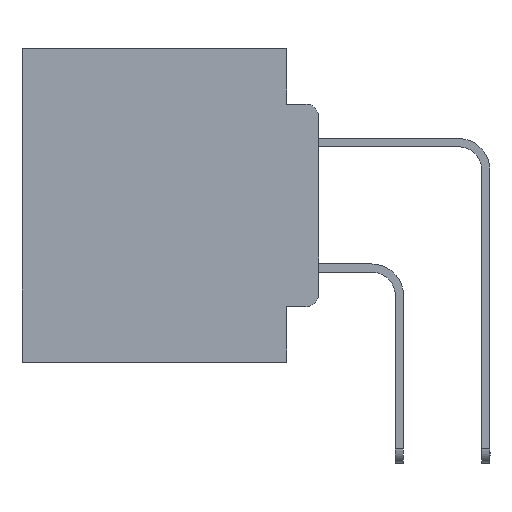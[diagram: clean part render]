
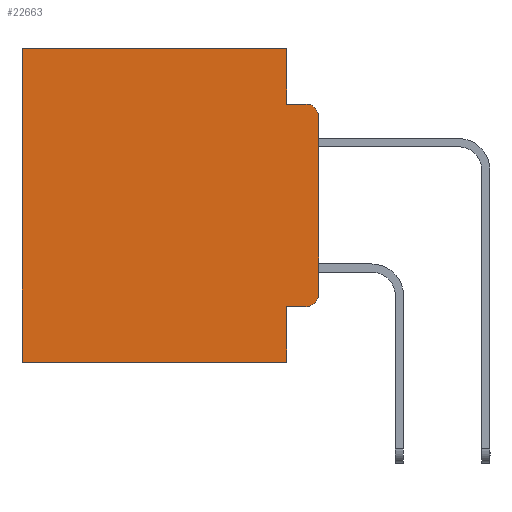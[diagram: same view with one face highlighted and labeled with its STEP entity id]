
A CAD part, left-side view. The second image highlights one B-rep face of the part: STEP entity #22663.
In plain terms, the highlighted planar face has unit normal (-1, 0, 0).
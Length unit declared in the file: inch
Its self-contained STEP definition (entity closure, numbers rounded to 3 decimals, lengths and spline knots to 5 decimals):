
#62 = EDGE_CURVE ( 'NONE', #12514, #3945, #13382, .T. ) ;
#63 = EDGE_LOOP ( 'NONE', ( #21769, #2561, #18959, #17731, #18588, #6089, #12443, #4766, #265, #25057 ) ) ;
#265 = ORIENTED_EDGE ( 'NONE', *, *, #27777, .T. ) ;
#346 = CARTESIAN_POINT ( 'NONE',  ( 0.298, 0.051, 0. ) ) ;
#623 = LINE ( 'NONE', #18278, #24192 ) ;
#1104 = PLANE ( 'NONE',  #4373 ) ;
#1684 = VECTOR ( 'NONE', #17175, 39.37008 ) ;
#1720 = DIRECTION ( 'NONE',  ( -1., 0., 0. ) ) ;
#1902 = LINE ( 'NONE', #10855, #5172 ) ;
#2036 = DIRECTION ( 'NONE',  ( -1., 0., 0. ) ) ;
#2121 = VERTEX_POINT ( 'NONE', #9627 ) ;
#2561 = ORIENTED_EDGE ( 'NONE', *, *, #25646, .T. ) ;
#2617 = EDGE_CURVE ( 'NONE', #12514, #18378, #17990, .T. ) ;
#3945 = VERTEX_POINT ( 'NONE', #20756 ) ;
#4373 = AXIS2_PLACEMENT_3D ( 'NONE', #25403, #14542, #9936 ) ;
#4402 = CARTESIAN_POINT ( 'NONE',  ( 0.298, 0.02, -0.4115 ) ) ;
#4596 = CARTESIAN_POINT ( 'NONE',  ( 0.298, 0.473, 0. ) ) ;
#4766 = ORIENTED_EDGE ( 'NONE', *, *, #17363, .F. ) ;
#5102 = CARTESIAN_POINT ( 'NONE',  ( 0.298, 0.051, -0.0885 ) ) ;
#5162 = CARTESIAN_POINT ( 'NONE',  ( 0.298, 0.051, -0.4115 ) ) ;
#5172 = VECTOR ( 'NONE', #25903, 39.37008 ) ;
#5721 = CIRCLE ( 'NONE', #9902, 0.02 ) ;
#5852 = VECTOR ( 'NONE', #24654, 39.37008 ) ;
#5875 = VECTOR ( 'NONE', #18188, 39.37008 ) ;
#6089 = ORIENTED_EDGE ( 'NONE', *, *, #8888, .T. ) ;
#6342 = CARTESIAN_POINT ( 'NONE',  ( 0.298, 0.02, -0.1085 ) ) ;
#6419 = VECTOR ( 'NONE', #6454, 39.37008 ) ;
#6454 = DIRECTION ( 'NONE',  ( 0., 1., 0. ) ) ;
#6927 = LINE ( 'NONE', #5162, #5875 ) ;
#7237 = LINE ( 'NONE', #7379, #23154 ) ;
#7301 = DIRECTION ( 'NONE',  ( 0., 0., -1. ) ) ;
#7379 = CARTESIAN_POINT ( 'NONE',  ( 0.298, 0., -0.5 ) ) ;
#8370 = CARTESIAN_POINT ( 'NONE',  ( 0.298, 0.051, -0.0885 ) ) ;
#8377 = DIRECTION ( 'NONE',  ( 0., 0., -1. ) ) ;
#8888 = EDGE_CURVE ( 'NONE', #3945, #11539, #23809, .T. ) ;
#9115 = VERTEX_POINT ( 'NONE', #21038 ) ;
#9627 = CARTESIAN_POINT ( 'NONE',  ( 0.298, 0., -0.1085 ) ) ;
#9902 = AXIS2_PLACEMENT_3D ( 'NONE', #13582, #2036, #17627 ) ;
#9936 = DIRECTION ( 'NONE',  ( 0., 0., -1. ) ) ;
#10855 = CARTESIAN_POINT ( 'NONE',  ( 0.298, 0.051, 0. ) ) ;
#10905 = VERTEX_POINT ( 'NONE', #4402 ) ;
#11539 = VERTEX_POINT ( 'NONE', #15780 ) ;
#11843 = VERTEX_POINT ( 'NONE', #24680 ) ;
#12443 = ORIENTED_EDGE ( 'NONE', *, *, #17432, .F. ) ;
#12514 = VERTEX_POINT ( 'NONE', #17100 ) ;
#12809 = CARTESIAN_POINT ( 'NONE',  ( 0.298, 0., 0. ) ) ;
#13382 = LINE ( 'NONE', #12809, #6419 ) ;
#13582 = CARTESIAN_POINT ( 'NONE',  ( 0.298, 0.02, -0.3915 ) ) ;
#14542 = DIRECTION ( 'NONE',  ( 1., 0., 0. ) ) ;
#14545 = VECTOR ( 'NONE', #17297, 39.37008 ) ;
#15626 = DIRECTION ( 'NONE',  ( 0., 1., 0. ) ) ;
#15780 = CARTESIAN_POINT ( 'NONE',  ( 0.298, 0.473, -0.5 ) ) ;
#16989 = VERTEX_POINT ( 'NONE', #26488 ) ;
#17100 = CARTESIAN_POINT ( 'NONE',  ( 0.298, 0.051, 0. ) ) ;
#17175 = DIRECTION ( 'NONE',  ( 0., -1., 0. ) ) ;
#17297 = DIRECTION ( 'NONE',  ( 0., 0., -1. ) ) ;
#17363 = EDGE_CURVE ( 'NONE', #16989, #23591, #1902, .T. ) ;
#17432 = EDGE_CURVE ( 'NONE', #23591, #11539, #7237, .T. ) ;
#17627 = DIRECTION ( 'NONE',  ( 0., 0., -1. ) ) ;
#17731 = ORIENTED_EDGE ( 'NONE', *, *, #2617, .F. ) ;
#17990 = LINE ( 'NONE', #346, #5852 ) ;
#18188 = DIRECTION ( 'NONE',  ( 0., -1., 0. ) ) ;
#18278 = CARTESIAN_POINT ( 'NONE',  ( 0.298, 0., 0. ) ) ;
#18378 = VERTEX_POINT ( 'NONE', #5102 ) ;
#18588 = ORIENTED_EDGE ( 'NONE', *, *, #62, .T. ) ;
#18959 = ORIENTED_EDGE ( 'NONE', *, *, #24391, .F. ) ;
#19781 = CIRCLE ( 'NONE', #23922, 0.02 ) ;
#20023 = EDGE_CURVE ( 'NONE', #2121, #11843, #623, .T. ) ;
#20756 = CARTESIAN_POINT ( 'NONE',  ( 0.298, 0.473, 0. ) ) ;
#21038 = CARTESIAN_POINT ( 'NONE',  ( 0.298, 0.02, -0.0885 ) ) ;
#21769 = ORIENTED_EDGE ( 'NONE', *, *, #20023, .F. ) ;
#22009 = EDGE_CURVE ( 'NONE', #10905, #11843, #5721, .T. ) ;
#22663 = ADVANCED_FACE ( 'NONE', ( #23510 ), #1104, .F. ) ;
#22718 = CARTESIAN_POINT ( 'NONE',  ( 0.298, 0.051, -0.5 ) ) ;
#23154 = VECTOR ( 'NONE', #15626, 39.37008 ) ;
#23510 = FACE_OUTER_BOUND ( 'NONE', #63, .T. ) ;
#23591 = VERTEX_POINT ( 'NONE', #22718 ) ;
#23809 = LINE ( 'NONE', #4596, #14545 ) ;
#23922 = AXIS2_PLACEMENT_3D ( 'NONE', #6342, #1720, #8377 ) ;
#24192 = VECTOR ( 'NONE', #7301, 39.37008 ) ;
#24391 = EDGE_CURVE ( 'NONE', #18378, #9115, #28163, .T. ) ;
#24654 = DIRECTION ( 'NONE',  ( 0., 0., -1. ) ) ;
#24680 = CARTESIAN_POINT ( 'NONE',  ( 0.298, 0., -0.3915 ) ) ;
#25057 = ORIENTED_EDGE ( 'NONE', *, *, #22009, .T. ) ;
#25403 = CARTESIAN_POINT ( 'NONE',  ( 0.298, 0., 0. ) ) ;
#25646 = EDGE_CURVE ( 'NONE', #2121, #9115, #19781, .T. ) ;
#25903 = DIRECTION ( 'NONE',  ( 0., 0., -1. ) ) ;
#26488 = CARTESIAN_POINT ( 'NONE',  ( 0.298, 0.051, -0.4115 ) ) ;
#27777 = EDGE_CURVE ( 'NONE', #16989, #10905, #6927, .T. ) ;
#28163 = LINE ( 'NONE', #8370, #1684 ) ;
